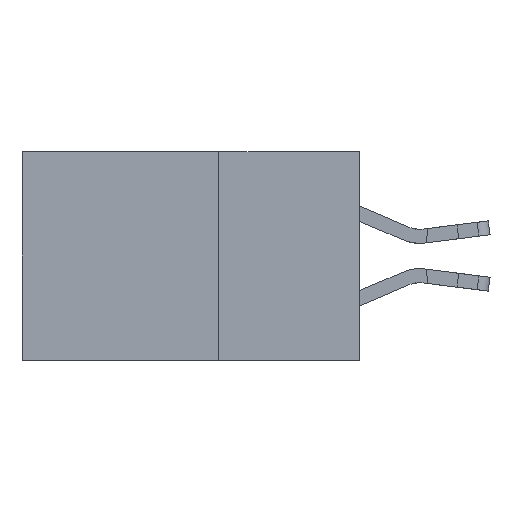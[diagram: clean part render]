
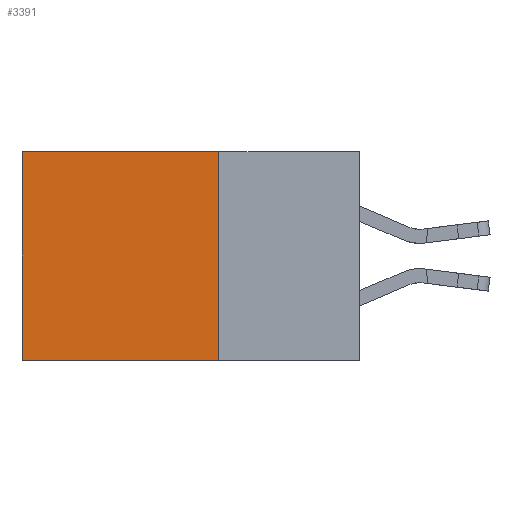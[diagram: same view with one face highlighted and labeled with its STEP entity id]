
A CAD part, left-side view. The second image highlights one B-rep face of the part: STEP entity #3391.
In plain terms, the highlighted planar face has unit normal (-1, 0, 0).
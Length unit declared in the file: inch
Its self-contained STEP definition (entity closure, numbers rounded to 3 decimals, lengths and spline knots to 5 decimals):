
#157 = EDGE_CURVE ( 'NONE', #16120, #5799, #34088, .T. ) ;
#2268 = VECTOR ( 'NONE', #29630, 39.37008 ) ;
#3391 = ADVANCED_FACE ( 'NONE', ( #8217 ), #25951, .F. ) ;
#4318 = CARTESIAN_POINT ( 'NONE',  ( 0.2875, 0.25, 0. ) ) ;
#4579 = EDGE_CURVE ( 'NONE', #9060, #16120, #13525, .T. ) ;
#5467 = ORIENTED_EDGE ( 'NONE', *, *, #157, .F. ) ;
#5606 = CARTESIAN_POINT ( 'NONE',  ( 0.2875, 0.6, 0. ) ) ;
#5799 = VERTEX_POINT ( 'NONE', #30897 ) ;
#6862 = EDGE_CURVE ( 'NONE', #9060, #20541, #15494, .T. ) ;
#7025 = DIRECTION ( 'NONE',  ( 0., 0., -1. ) ) ;
#8217 = FACE_OUTER_BOUND ( 'NONE', #33085, .T. ) ;
#8867 = DIRECTION ( 'NONE',  ( 0., 1., 0. ) ) ;
#9060 = VERTEX_POINT ( 'NONE', #34259 ) ;
#9929 = VECTOR ( 'NONE', #19151, 39.37008 ) ;
#13235 = ORIENTED_EDGE ( 'NONE', *, *, #6862, .T. ) ;
#13525 = LINE ( 'NONE', #13773, #2268 ) ;
#13773 = CARTESIAN_POINT ( 'NONE',  ( 0.2875, 0.25, 0. ) ) ;
#15494 = LINE ( 'NONE', #24883, #28813 ) ;
#16120 = VERTEX_POINT ( 'NONE', #33108 ) ;
#16449 = CARTESIAN_POINT ( 'NONE',  ( 0.2875, 0.6, 0. ) ) ;
#18105 = DIRECTION ( 'NONE',  ( 1., 0., 0. ) ) ;
#19151 = DIRECTION ( 'NONE',  ( 0., 0., -1. ) ) ;
#19438 = EDGE_CURVE ( 'NONE', #20541, #5799, #33674, .T. ) ;
#20541 = VERTEX_POINT ( 'NONE', #5606 ) ;
#23748 = ORIENTED_EDGE ( 'NONE', *, *, #4579, .F. ) ;
#24883 = CARTESIAN_POINT ( 'NONE',  ( 0.2875, 0.25, 0. ) ) ;
#25096 = AXIS2_PLACEMENT_3D ( 'NONE', #4318, #18105, #7025 ) ;
#25647 = ORIENTED_EDGE ( 'NONE', *, *, #19438, .T. ) ;
#25951 = PLANE ( 'NONE',  #25096 ) ;
#26663 = VECTOR ( 'NONE', #29145, 39.37008 ) ;
#28813 = VECTOR ( 'NONE', #8867, 39.37008 ) ;
#29145 = DIRECTION ( 'NONE',  ( 0., 1., 0. ) ) ;
#29630 = DIRECTION ( 'NONE',  ( 0., 0., -1. ) ) ;
#30897 = CARTESIAN_POINT ( 'NONE',  ( 0.2875, 0.6, -0.37 ) ) ;
#31375 = CARTESIAN_POINT ( 'NONE',  ( 0.2875, 0.25, -0.37 ) ) ;
#33085 = EDGE_LOOP ( 'NONE', ( #25647, #5467, #23748, #13235 ) ) ;
#33108 = CARTESIAN_POINT ( 'NONE',  ( 0.2875, 0.25, -0.37 ) ) ;
#33674 = LINE ( 'NONE', #16449, #9929 ) ;
#34088 = LINE ( 'NONE', #31375, #26663 ) ;
#34259 = CARTESIAN_POINT ( 'NONE',  ( 0.2875, 0.25, 0. ) ) ;
